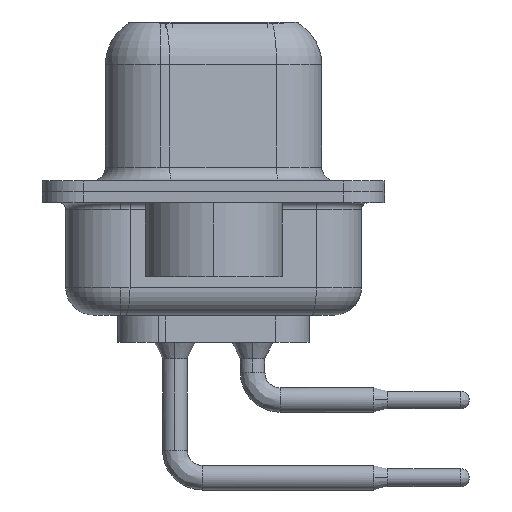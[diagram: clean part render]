
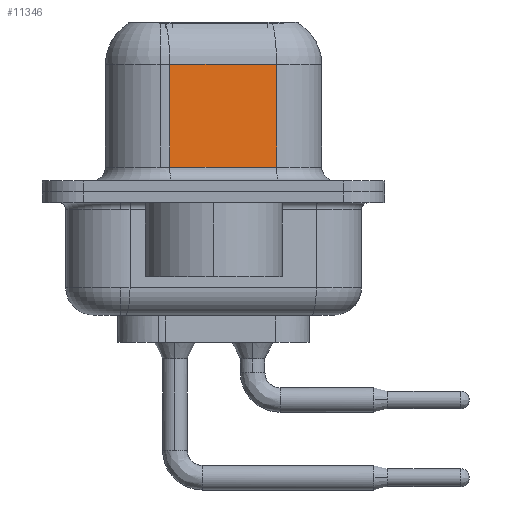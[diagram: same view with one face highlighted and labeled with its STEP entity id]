
A CAD part, left-side view. The second image highlights one B-rep face of the part: STEP entity #11346.
In plain terms, the highlighted planar face has unit normal (-0.985, -0.174, 0).
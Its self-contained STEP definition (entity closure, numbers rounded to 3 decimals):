
#345 = DIRECTION ( 'NONE',  ( 0.985, 0.174, 0. ) ) ;
#752 = LINE ( 'NONE', #21977, #18290 ) ;
#984 = ORIENTED_EDGE ( 'NONE', *, *, #15296, .T. ) ;
#1700 = FACE_OUTER_BOUND ( 'NONE', #8965, .T. ) ;
#1849 = VERTEX_POINT ( 'NONE', #12566 ) ;
#2622 = LINE ( 'NONE', #20907, #20070 ) ;
#4048 = LINE ( 'NONE', #15814, #20997 ) ;
#4262 = LINE ( 'NONE', #9658, #12697 ) ;
#6488 = ORIENTED_EDGE ( 'NONE', *, *, #20327, .T. ) ;
#6735 = ORIENTED_EDGE ( 'NONE', *, *, #7360, .F. ) ;
#7360 = EDGE_CURVE ( 'NONE', #20382, #1849, #2622, .T. ) ;
#7720 = DIRECTION ( 'NONE',  ( -0.174, 0.985, 0. ) ) ;
#8965 = EDGE_LOOP ( 'NONE', ( #6735, #16909, #984, #6488 ) ) ;
#9658 = CARTESIAN_POINT ( 'NONE',  ( 5.043, -2.297, 0.9 ) ) ;
#10525 = CARTESIAN_POINT ( 'NONE',  ( 5.043, -2.297, 6.4 ) ) ;
#11346 = ADVANCED_FACE ( 'NONE', ( #1700 ), #15554, .F. ) ;
#12211 = DIRECTION ( 'NONE',  ( -0.174, 0.985, 0. ) ) ;
#12426 = DIRECTION ( 'NONE',  ( 0., 0., -1. ) ) ;
#12566 = CARTESIAN_POINT ( 'NONE',  ( 5.043, -2.297, 0.9 ) ) ;
#12697 = VECTOR ( 'NONE', #16492, 1000. ) ;
#13432 = EDGE_CURVE ( 'NONE', #20382, #14094, #4048, .T. ) ;
#13486 = DIRECTION ( 'NONE',  ( 0., 0., -1. ) ) ;
#14069 = AXIS2_PLACEMENT_3D ( 'NONE', #10525, #345, #12211 ) ;
#14094 = VERTEX_POINT ( 'NONE', #16230 ) ;
#14762 = VERTEX_POINT ( 'NONE', #19618 ) ;
#15296 = EDGE_CURVE ( 'NONE', #14094, #14762, #752, .T. ) ;
#15554 = PLANE ( 'NONE',  #14069 ) ;
#15814 = CARTESIAN_POINT ( 'NONE',  ( 5.043, -2.297, 4.65 ) ) ;
#16230 = CARTESIAN_POINT ( 'NONE',  ( 4.355, 1.603, 4.65 ) ) ;
#16492 = DIRECTION ( 'NONE',  ( 0.174, -0.985, 0. ) ) ;
#16568 = CARTESIAN_POINT ( 'NONE',  ( 5.043, -2.297, 4.65 ) ) ;
#16909 = ORIENTED_EDGE ( 'NONE', *, *, #13432, .T. ) ;
#18290 = VECTOR ( 'NONE', #13486, 1000. ) ;
#19618 = CARTESIAN_POINT ( 'NONE',  ( 4.355, 1.603, 0.9 ) ) ;
#20070 = VECTOR ( 'NONE', #12426, 1000. ) ;
#20327 = EDGE_CURVE ( 'NONE', #14762, #1849, #4262, .T. ) ;
#20382 = VERTEX_POINT ( 'NONE', #16568 ) ;
#20907 = CARTESIAN_POINT ( 'NONE',  ( 5.043, -2.297, 6.4 ) ) ;
#20997 = VECTOR ( 'NONE', #7720, 1000. ) ;
#21977 = CARTESIAN_POINT ( 'NONE',  ( 4.355, 1.603, 6.4 ) ) ;
